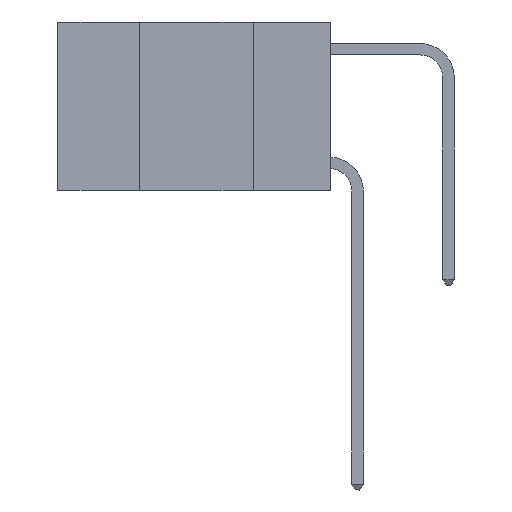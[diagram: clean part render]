
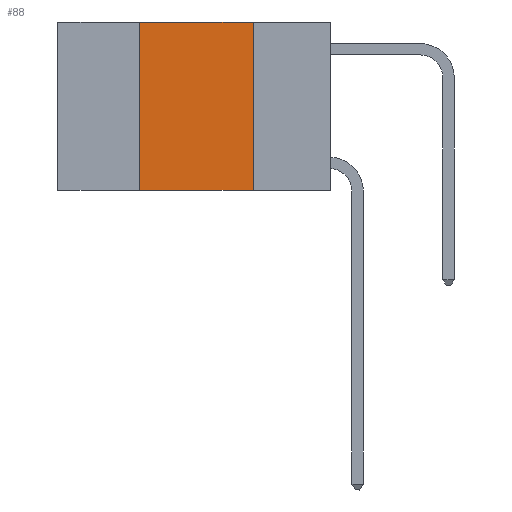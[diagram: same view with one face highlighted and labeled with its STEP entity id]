
A CAD part, left-side view. The second image highlights one B-rep face of the part: STEP entity #88.
In plain terms, the highlighted planar face has unit normal (-1, 0, 0).
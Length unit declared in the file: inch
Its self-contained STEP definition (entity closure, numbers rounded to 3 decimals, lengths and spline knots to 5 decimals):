
#73 = CARTESIAN_POINT ( 'NONE',  ( 0., 0.17, -0.37 ) ) ;
#88 = ADVANCED_FACE ( 'NONE', ( #19443 ), #25025, .F. ) ;
#491 = ORIENTED_EDGE ( 'NONE', *, *, #18281, .F. ) ;
#1385 = CARTESIAN_POINT ( 'NONE',  ( 0., 0.42, 0. ) ) ;
#2380 = LINE ( 'NONE', #10346, #6964 ) ;
#3057 = VECTOR ( 'NONE', #15762, 39.37008 ) ;
#3446 = VECTOR ( 'NONE', #23401, 39.37008 ) ;
#4979 = EDGE_CURVE ( 'NONE', #6713, #5421, #13466, .T. ) ;
#5421 = VERTEX_POINT ( 'NONE', #1385 ) ;
#6276 = ORIENTED_EDGE ( 'NONE', *, *, #20858, .F. ) ;
#6713 = VERTEX_POINT ( 'NONE', #7373 ) ;
#6964 = VECTOR ( 'NONE', #8383, 39.37008 ) ;
#7373 = CARTESIAN_POINT ( 'NONE',  ( 0., 0.42, -0.37 ) ) ;
#8383 = DIRECTION ( 'NONE',  ( 0., 0., -1. ) ) ;
#8623 = CARTESIAN_POINT ( 'NONE',  ( 0., 0.6, 0. ) ) ;
#8858 = CARTESIAN_POINT ( 'NONE',  ( 0., 0.17, 0. ) ) ;
#8865 = CARTESIAN_POINT ( 'NONE',  ( 0., 0.6, -0.37 ) ) ;
#8896 = LINE ( 'NONE', #8865, #23858 ) ;
#10346 = CARTESIAN_POINT ( 'NONE',  ( 0., 0.17, 0. ) ) ;
#11040 = DIRECTION ( 'NONE',  ( 0., 0., -1. ) ) ;
#11462 = ORIENTED_EDGE ( 'NONE', *, *, #4979, .F. ) ;
#13459 = AXIS2_PLACEMENT_3D ( 'NONE', #8623, #23978, #11040 ) ;
#13466 = LINE ( 'NONE', #13809, #3057 ) ;
#13809 = CARTESIAN_POINT ( 'NONE',  ( 0., 0.42, 0. ) ) ;
#13869 = LINE ( 'NONE', #21468, #3446 ) ;
#15546 = EDGE_LOOP ( 'NONE', ( #491, #6276, #11462, #16689 ) ) ;
#15762 = DIRECTION ( 'NONE',  ( 0., 0., 1. ) ) ;
#16689 = ORIENTED_EDGE ( 'NONE', *, *, #21956, .T. ) ;
#18281 = EDGE_CURVE ( 'NONE', #24919, #22265, #2380, .T. ) ;
#19443 = FACE_OUTER_BOUND ( 'NONE', #15546, .T. ) ;
#20591 = DIRECTION ( 'NONE',  ( 0., -1., 0. ) ) ;
#20858 = EDGE_CURVE ( 'NONE', #5421, #24919, #13869, .T. ) ;
#21468 = CARTESIAN_POINT ( 'NONE',  ( 0., 0.6, 0. ) ) ;
#21956 = EDGE_CURVE ( 'NONE', #6713, #22265, #8896, .T. ) ;
#22265 = VERTEX_POINT ( 'NONE', #73 ) ;
#23401 = DIRECTION ( 'NONE',  ( 0., -1., 0. ) ) ;
#23858 = VECTOR ( 'NONE', #20591, 39.37008 ) ;
#23978 = DIRECTION ( 'NONE',  ( 1., 0., 0. ) ) ;
#24919 = VERTEX_POINT ( 'NONE', #8858 ) ;
#25025 = PLANE ( 'NONE',  #13459 ) ;
